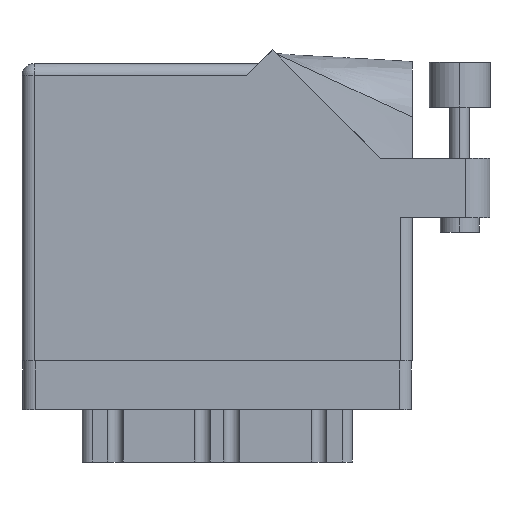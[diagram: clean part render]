
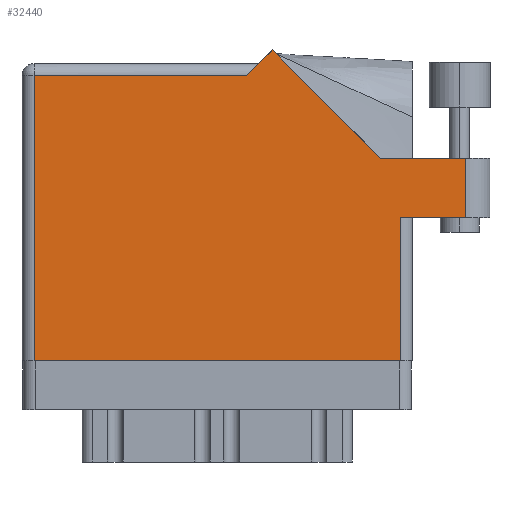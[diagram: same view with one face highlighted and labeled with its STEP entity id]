
A CAD part, front view. The second image highlights one B-rep face of the part: STEP entity #32440.
In plain terms, the highlighted face is planar.
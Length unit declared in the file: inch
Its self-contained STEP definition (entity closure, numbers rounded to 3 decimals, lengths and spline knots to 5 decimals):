
#357 = DIRECTION ( 'NONE',  ( -1., 0., 0. ) ) ;
#693 = ORIENTED_EDGE ( 'NONE', *, *, #24549, .T. ) ;
#1156 = ORIENTED_EDGE ( 'NONE', *, *, #4782, .T. ) ;
#1263 = CARTESIAN_POINT ( 'NONE',  ( 1.217, 1.53, 0. ) ) ;
#2057 = FACE_OUTER_BOUND ( 'NONE', #28116, .T. ) ;
#2117 = VERTEX_POINT ( 'NONE', #26090 ) ;
#2610 = ORIENTED_EDGE ( 'NONE', *, *, #33374, .T. ) ;
#2727 = DIRECTION ( 'NONE',  ( 1., 0., 0. ) ) ;
#2844 = CARTESIAN_POINT ( 'NONE',  ( 2.285, 1.044, 0. ) ) ;
#3031 = CARTESIAN_POINT ( 'NONE',  ( 2.41, 1.044, 0. ) ) ;
#3844 = ORIENTED_EDGE ( 'NONE', *, *, #12551, .T. ) ;
#4782 = EDGE_CURVE ( 'NONE', #23823, #15078, #9954, .T. ) ;
#5050 = DIRECTION ( 'NONE',  ( -1., 0., 0. ) ) ;
#5394 = CARTESIAN_POINT ( 'NONE',  ( 1.948, 0.737, 0. ) ) ;
#7009 = VECTOR ( 'NONE', #21167, 39.37008 ) ;
#7961 = CARTESIAN_POINT ( 'NONE',  ( 1.948, 0.737, 0. ) ) ;
#8180 = CARTESIAN_POINT ( 'NONE',  ( 0.062, 0., 0. ) ) ;
#8339 = CARTESIAN_POINT ( 'NONE',  ( 1.84442, 1.044, 0. ) ) ;
#9493 = EDGE_CURVE ( 'NONE', #15078, #31311, #10780, .T. ) ;
#9816 = CARTESIAN_POINT ( 'NONE',  ( 0., 1.53, 0. ) ) ;
#9954 = LINE ( 'NONE', #21044, #15401 ) ;
#10780 = LINE ( 'NONE', #7961, #7009 ) ;
#12551 = EDGE_CURVE ( 'NONE', #32129, #33935, #34699, .T. ) ;
#14290 = DIRECTION ( 'NONE',  ( -0.707, -0.707, 0. ) ) ;
#14546 = DIRECTION ( 'NONE',  ( 0., 1., 0. ) ) ;
#14836 = CARTESIAN_POINT ( 'NONE',  ( 1.28771, 1.60071, 0. ) ) ;
#14883 = EDGE_CURVE ( 'NONE', #2117, #15409, #21676, .T. ) ;
#15078 = VERTEX_POINT ( 'NONE', #25820 ) ;
#15401 = VECTOR ( 'NONE', #2727, 39.37008 ) ;
#15409 = VERTEX_POINT ( 'NONE', #27404 ) ;
#15703 = VECTOR ( 'NONE', #14290, 39.37008 ) ;
#16338 = CARTESIAN_POINT ( 'NONE',  ( 1.155, 1.468, 0. ) ) ;
#16395 = LINE ( 'NONE', #3031, #16725 ) ;
#16725 = VECTOR ( 'NONE', #34560, 39.37008 ) ;
#16786 = VECTOR ( 'NONE', #14546, 39.37008 ) ;
#18139 = DIRECTION ( 'NONE',  ( 1., 0., 0. ) ) ;
#18228 = VECTOR ( 'NONE', #18139, 39.37008 ) ;
#18644 = EDGE_CURVE ( 'NONE', #33935, #23823, #26170, .T. ) ;
#19138 = VECTOR ( 'NONE', #34093, 39.37008 ) ;
#20345 = VECTOR ( 'NONE', #32307, 39.37008 ) ;
#20440 = VECTOR ( 'NONE', #357, 39.37008 ) ;
#20547 = PLANE ( 'NONE',  #28487 ) ;
#20677 = ORIENTED_EDGE ( 'NONE', *, *, #18644, .T. ) ;
#20864 = ORIENTED_EDGE ( 'NONE', *, *, #14883, .T. ) ;
#20951 = CARTESIAN_POINT ( 'NONE',  ( 2.01, 0.737, 0. ) ) ;
#21044 = CARTESIAN_POINT ( 'NONE',  ( 0., 0., 0. ) ) ;
#21167 = DIRECTION ( 'NONE',  ( 0., 1., 0. ) ) ;
#21380 = LINE ( 'NONE', #8339, #20345 ) ;
#21676 = LINE ( 'NONE', #2844, #16786 ) ;
#23047 = ORIENTED_EDGE ( 'NONE', *, *, #29051, .T. ) ;
#23230 = LINE ( 'NONE', #20951, #18228 ) ;
#23364 = VERTEX_POINT ( 'NONE', #24578 ) ;
#23694 = DIRECTION ( 'NONE',  ( 0., 0., -1. ) ) ;
#23823 = VERTEX_POINT ( 'NONE', #8180 ) ;
#24549 = EDGE_CURVE ( 'NONE', #31311, #2117, #23230, .T. ) ;
#24578 = CARTESIAN_POINT ( 'NONE',  ( 1.84442, 1.044, 0. ) ) ;
#25183 = VERTEX_POINT ( 'NONE', #14836 ) ;
#25820 = CARTESIAN_POINT ( 'NONE',  ( 1.948, 0., 0. ) ) ;
#26090 = CARTESIAN_POINT ( 'NONE',  ( 2.285, 0.737, 0. ) ) ;
#26170 = LINE ( 'NONE', #26343, #19138 ) ;
#26336 = EDGE_CURVE ( 'NONE', #25183, #32129, #27678, .T. ) ;
#26343 = CARTESIAN_POINT ( 'NONE',  ( 0.062, 0., 0. ) ) ;
#27404 = CARTESIAN_POINT ( 'NONE',  ( 2.285, 1.044, 0. ) ) ;
#27678 = LINE ( 'NONE', #1263, #15703 ) ;
#28116 = EDGE_LOOP ( 'NONE', ( #693, #20864, #2610, #23047, #28238, #3844, #20677, #1156, #31857 ) ) ;
#28238 = ORIENTED_EDGE ( 'NONE', *, *, #26336, .T. ) ;
#28487 = AXIS2_PLACEMENT_3D ( 'NONE', #9816, #23694, #5050 ) ;
#29051 = EDGE_CURVE ( 'NONE', #23364, #25183, #21380, .T. ) ;
#29418 = CARTESIAN_POINT ( 'NONE',  ( 0.062, 1.468, 0. ) ) ;
#29589 = CARTESIAN_POINT ( 'NONE',  ( 0., 1.468, 0. ) ) ;
#31311 = VERTEX_POINT ( 'NONE', #5394 ) ;
#31857 = ORIENTED_EDGE ( 'NONE', *, *, #9493, .T. ) ;
#32129 = VERTEX_POINT ( 'NONE', #16338 ) ;
#32307 = DIRECTION ( 'NONE',  ( -0.707, 0.707, 0. ) ) ;
#32440 = ADVANCED_FACE ( 'NONE', ( #2057 ), #20547, .F. ) ;
#33374 = EDGE_CURVE ( 'NONE', #15409, #23364, #16395, .T. ) ;
#33935 = VERTEX_POINT ( 'NONE', #29418 ) ;
#34093 = DIRECTION ( 'NONE',  ( 0., -1., 0. ) ) ;
#34560 = DIRECTION ( 'NONE',  ( -1., 0., 0. ) ) ;
#34699 = LINE ( 'NONE', #29589, #20440 ) ;
